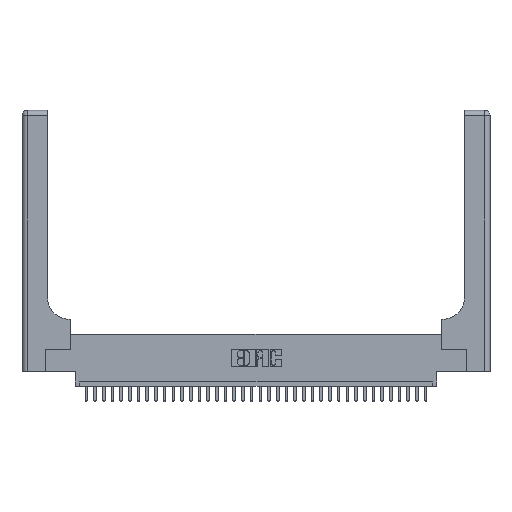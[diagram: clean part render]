
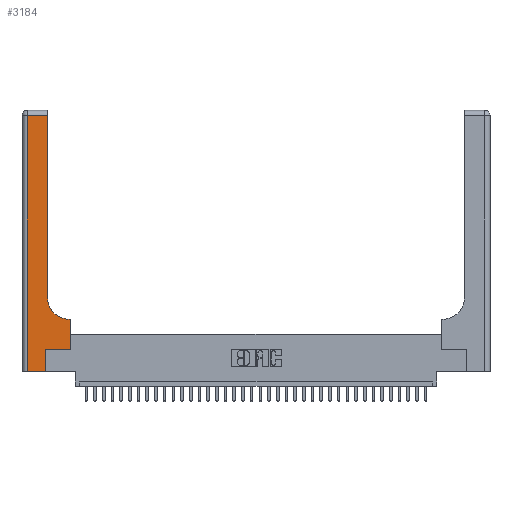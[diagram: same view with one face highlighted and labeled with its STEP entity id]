
A CAD part, top view. The second image highlights one B-rep face of the part: STEP entity #3184.
In plain terms, the highlighted planar face has unit normal (0, 0, 1).
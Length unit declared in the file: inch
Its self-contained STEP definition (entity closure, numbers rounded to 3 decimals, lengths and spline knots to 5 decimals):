
#49 = EDGE_CURVE ( 'NONE', #14884, #30987, #35028, .T. ) ;
#69 = CARTESIAN_POINT ( 'NONE',  ( 0., 3., 0.37 ) ) ;
#276 = DIRECTION ( 'NONE',  ( 1., 0., 0. ) ) ;
#1269 = CARTESIAN_POINT ( 'NONE',  ( 0.5585, 0.6, 0.37 ) ) ;
#1341 = DIRECTION ( 'NONE',  ( 0., 1., 0. ) ) ;
#1523 = LINE ( 'NONE', #17479, #12317 ) ;
#1785 = ORIENTED_EDGE ( 'NONE', *, *, #21443, .T. ) ;
#3184 = ADVANCED_FACE ( 'NONE', ( #34944 ), #27558, .F. ) ;
#3332 = CARTESIAN_POINT ( 'NONE',  ( 0.5585, 0.25, 0.37 ) ) ;
#5619 = DIRECTION ( 'NONE',  ( 0., 0., -1. ) ) ;
#5984 = EDGE_CURVE ( 'NONE', #9151, #22756, #20417, .T. ) ;
#6280 = CARTESIAN_POINT ( 'NONE',  ( 0.5415, 0.85, 0.37 ) ) ;
#6454 = DIRECTION ( 'NONE',  ( 0., 1., 0. ) ) ;
#7143 = ORIENTED_EDGE ( 'NONE', *, *, #49, .T. ) ;
#8776 = AXIS2_PLACEMENT_3D ( 'NONE', #69, #5619, #19357 ) ;
#9151 = VERTEX_POINT ( 'NONE', #12021 ) ;
#9401 = DIRECTION ( 'NONE',  ( 0., 0., -1. ) ) ;
#10561 = DIRECTION ( 'NONE',  ( -1., 0., 0. ) ) ;
#10804 = CARTESIAN_POINT ( 'NONE',  ( 0.2915, 0.6, 0.37 ) ) ;
#10808 = VECTOR ( 'NONE', #10561, 39.37008 ) ;
#11381 = DIRECTION ( 'NONE',  ( 0., -1., 0. ) ) ;
#11551 = VECTOR ( 'NONE', #276, 39.37008 ) ;
#11559 = ORIENTED_EDGE ( 'NONE', *, *, #17403, .T. ) ;
#11862 = CARTESIAN_POINT ( 'NONE',  ( 0.269, 0.25, 0.37 ) ) ;
#12021 = CARTESIAN_POINT ( 'NONE',  ( 0.06, 2.94, 0.37 ) ) ;
#12317 = VECTOR ( 'NONE', #1341, 39.37008 ) ;
#14404 = CARTESIAN_POINT ( 'NONE',  ( 0.2915, 3., 0.37 ) ) ;
#14568 = LINE ( 'NONE', #31342, #21856 ) ;
#14884 = VERTEX_POINT ( 'NONE', #31670 ) ;
#15828 = AXIS2_PLACEMENT_3D ( 'NONE', #6280, #9401, #25786 ) ;
#17286 = LINE ( 'NONE', #10804, #10808 ) ;
#17403 = EDGE_CURVE ( 'NONE', #22756, #33193, #34028, .T. ) ;
#17479 = CARTESIAN_POINT ( 'NONE',  ( 0.269, 0., 0.37 ) ) ;
#17870 = CARTESIAN_POINT ( 'NONE',  ( 0.2915, 2.94, 0.37 ) ) ;
#18274 = VERTEX_POINT ( 'NONE', #29324 ) ;
#18419 = VECTOR ( 'NONE', #6454, 39.37008 ) ;
#19140 = EDGE_CURVE ( 'NONE', #33193, #28152, #1523, .T. ) ;
#19357 = DIRECTION ( 'NONE',  ( -1., 0., 0. ) ) ;
#19578 = DIRECTION ( 'NONE',  ( 1., 0., 0. ) ) ;
#20078 = DIRECTION ( 'NONE',  ( -1., 0., 0. ) ) ;
#20278 = VECTOR ( 'NONE', #19578, 39.37008 ) ;
#20417 = LINE ( 'NONE', #27892, #26029 ) ;
#20723 = ORIENTED_EDGE ( 'NONE', *, *, #5984, .T. ) ;
#20750 = EDGE_LOOP ( 'NONE', ( #23035, #1785, #20723, #11559, #31358, #32601, #7143, #28447, #32115 ) ) ;
#21443 = EDGE_CURVE ( 'NONE', #28923, #9151, #14568, .T. ) ;
#21856 = VECTOR ( 'NONE', #20078, 39.37008 ) ;
#22079 = CARTESIAN_POINT ( 'NONE',  ( 0., 0., 0.37 ) ) ;
#22692 = LINE ( 'NONE', #14404, #18419 ) ;
#22756 = VERTEX_POINT ( 'NONE', #29427 ) ;
#23035 = ORIENTED_EDGE ( 'NONE', *, *, #28090, .T. ) ;
#23586 = DIRECTION ( 'NONE',  ( 0., 1., 0. ) ) ;
#24566 = LINE ( 'NONE', #27658, #20278 ) ;
#25786 = DIRECTION ( 'NONE',  ( 1., 0., 0. ) ) ;
#26029 = VECTOR ( 'NONE', #11381, 39.37008 ) ;
#26047 = EDGE_CURVE ( 'NONE', #28152, #14884, #24566, .T. ) ;
#26972 = EDGE_CURVE ( 'NONE', #27839, #18274, #32816, .T. ) ;
#27558 = PLANE ( 'NONE',  #8776 ) ;
#27658 = CARTESIAN_POINT ( 'NONE',  ( 0.269, 0.25, 0.37 ) ) ;
#27839 = VERTEX_POINT ( 'NONE', #30219 ) ;
#27892 = CARTESIAN_POINT ( 'NONE',  ( 0.06, 3., 0.37 ) ) ;
#28090 = EDGE_CURVE ( 'NONE', #18274, #28923, #22692, .T. ) ;
#28152 = VERTEX_POINT ( 'NONE', #11862 ) ;
#28447 = ORIENTED_EDGE ( 'NONE', *, *, #32304, .T. ) ;
#28923 = VERTEX_POINT ( 'NONE', #17870 ) ;
#29324 = CARTESIAN_POINT ( 'NONE',  ( 0.2915, 0.85, 0.37 ) ) ;
#29427 = CARTESIAN_POINT ( 'NONE',  ( 0.06, 0., 0.37 ) ) ;
#30219 = CARTESIAN_POINT ( 'NONE',  ( 0.5415, 0.6, 0.37 ) ) ;
#30987 = VERTEX_POINT ( 'NONE', #1269 ) ;
#31342 = CARTESIAN_POINT ( 'NONE',  ( 0., 2.94, 0.37 ) ) ;
#31358 = ORIENTED_EDGE ( 'NONE', *, *, #19140, .T. ) ;
#31519 = VECTOR ( 'NONE', #23586, 39.37008 ) ;
#31670 = CARTESIAN_POINT ( 'NONE',  ( 0.5585, 0.25, 0.37 ) ) ;
#32115 = ORIENTED_EDGE ( 'NONE', *, *, #26972, .T. ) ;
#32304 = EDGE_CURVE ( 'NONE', #30987, #27839, #17286, .T. ) ;
#32601 = ORIENTED_EDGE ( 'NONE', *, *, #26047, .T. ) ;
#32816 = CIRCLE ( 'NONE', #15828, 0.25 ) ;
#33193 = VERTEX_POINT ( 'NONE', #33604 ) ;
#33604 = CARTESIAN_POINT ( 'NONE',  ( 0.269, 0., 0.37 ) ) ;
#34028 = LINE ( 'NONE', #22079, #11551 ) ;
#34944 = FACE_OUTER_BOUND ( 'NONE', #20750, .T. ) ;
#35028 = LINE ( 'NONE', #3332, #31519 ) ;
